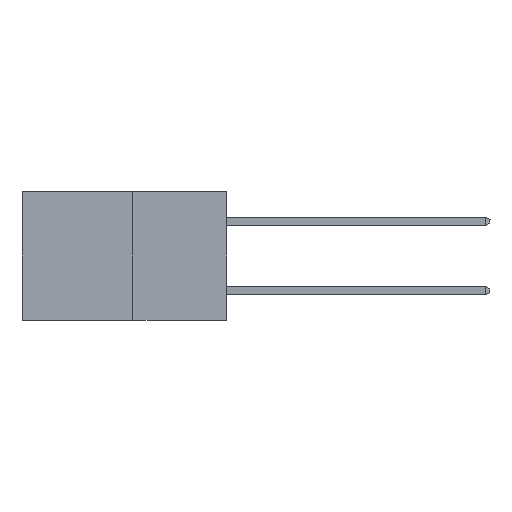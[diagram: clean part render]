
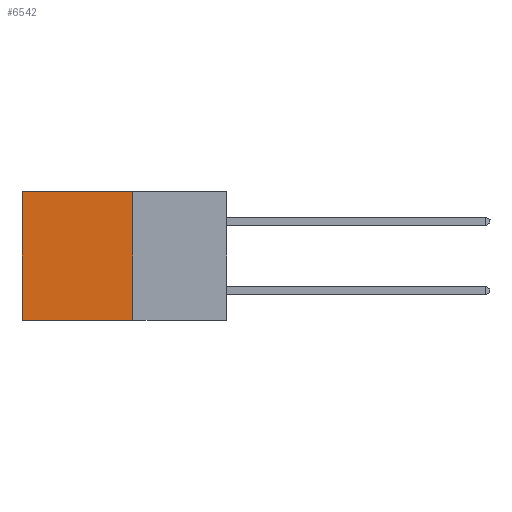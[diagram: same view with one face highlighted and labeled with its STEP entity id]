
A CAD part, left-side view. The second image highlights one B-rep face of the part: STEP entity #6542.
In plain terms, the highlighted planar face has unit normal (-1, 0, 0).
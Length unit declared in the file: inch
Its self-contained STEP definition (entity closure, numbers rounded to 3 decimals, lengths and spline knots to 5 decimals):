
#99 = LINE ( 'NONE', #5629, #1776 ) ;
#201 = CARTESIAN_POINT ( 'NONE',  ( 0.277, 0.27, 0. ) ) ;
#962 = ORIENTED_EDGE ( 'NONE', *, *, #3588, .F. ) ;
#1329 = CARTESIAN_POINT ( 'NONE',  ( 0.277, 0.59, -0.37 ) ) ;
#1346 = DIRECTION ( 'NONE',  ( 0., 1., 0. ) ) ;
#1451 = VECTOR ( 'NONE', #6985, 39.37008 ) ;
#1527 = CARTESIAN_POINT ( 'NONE',  ( 0.277, 0.27, 0. ) ) ;
#1529 = AXIS2_PLACEMENT_3D ( 'NONE', #2508, #2491, #2474 ) ;
#1776 = VECTOR ( 'NONE', #5915, 39.37008 ) ;
#2330 = CARTESIAN_POINT ( 'NONE',  ( 0.277, 0.59, -0.37 ) ) ;
#2474 = DIRECTION ( 'NONE',  ( 0., 0., -1. ) ) ;
#2491 = DIRECTION ( 'NONE',  ( 1., 0., 0. ) ) ;
#2508 = CARTESIAN_POINT ( 'NONE',  ( 0.277, 0.27, -0.37 ) ) ;
#2556 = PLANE ( 'NONE',  #1529 ) ;
#3243 = VERTEX_POINT ( 'NONE', #2330 ) ;
#3337 = ORIENTED_EDGE ( 'NONE', *, *, #7610, .F. ) ;
#3414 = CARTESIAN_POINT ( 'NONE',  ( 0.277, 0.59, 0. ) ) ;
#3588 = EDGE_CURVE ( 'NONE', #3638, #3243, #7931, .T. ) ;
#3638 = VERTEX_POINT ( 'NONE', #4090 ) ;
#4082 = EDGE_CURVE ( 'NONE', #7956, #8477, #7442, .T. ) ;
#4090 = CARTESIAN_POINT ( 'NONE',  ( 0.277, 0.27, -0.37 ) ) ;
#4249 = FACE_OUTER_BOUND ( 'NONE', #7966, .T. ) ;
#4530 = ORIENTED_EDGE ( 'NONE', *, *, #5472, .T. ) ;
#5101 = LINE ( 'NONE', #1329, #1451 ) ;
#5278 = ORIENTED_EDGE ( 'NONE', *, *, #4082, .T. ) ;
#5472 = EDGE_CURVE ( 'NONE', #8477, #3243, #5101, .T. ) ;
#5629 = CARTESIAN_POINT ( 'NONE',  ( 0.277, 0.27, -0.37 ) ) ;
#5726 = VECTOR ( 'NONE', #1346, 39.37008 ) ;
#5915 = DIRECTION ( 'NONE',  ( 0., 0., -1. ) ) ;
#6542 = ADVANCED_FACE ( 'NONE', ( #4249 ), #2556, .F. ) ;
#6985 = DIRECTION ( 'NONE',  ( 0., 0., -1. ) ) ;
#7442 = LINE ( 'NONE', #1527, #5726 ) ;
#7610 = EDGE_CURVE ( 'NONE', #7956, #3638, #99, .T. ) ;
#7740 = VECTOR ( 'NONE', #7900, 39.37008 ) ;
#7778 = CARTESIAN_POINT ( 'NONE',  ( 0.277, 0.27, -0.37 ) ) ;
#7900 = DIRECTION ( 'NONE',  ( 0., 1., 0. ) ) ;
#7931 = LINE ( 'NONE', #7778, #7740 ) ;
#7956 = VERTEX_POINT ( 'NONE', #201 ) ;
#7966 = EDGE_LOOP ( 'NONE', ( #4530, #962, #3337, #5278 ) ) ;
#8477 = VERTEX_POINT ( 'NONE', #3414 ) ;
